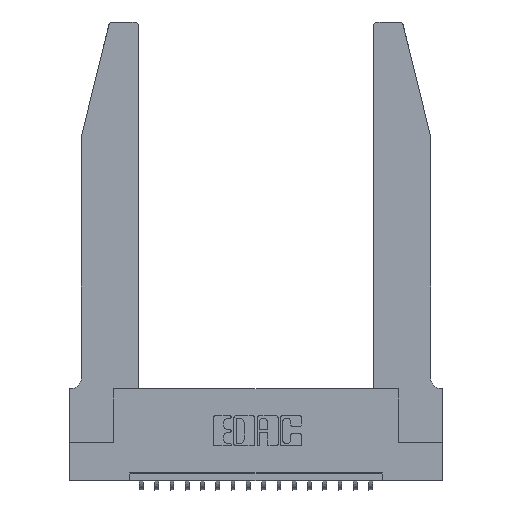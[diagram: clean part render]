
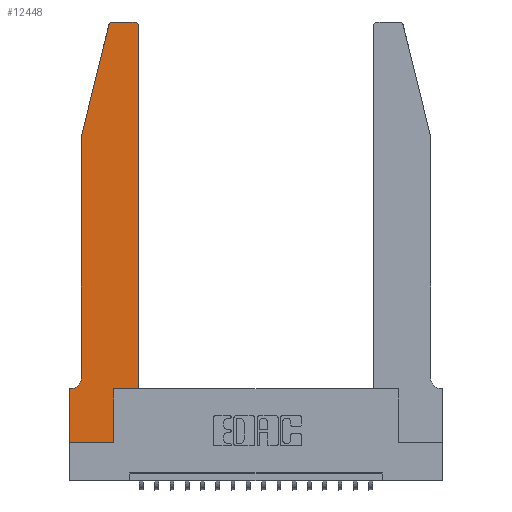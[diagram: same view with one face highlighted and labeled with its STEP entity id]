
A CAD part, top view. The second image highlights one B-rep face of the part: STEP entity #12448.
In plain terms, the highlighted planar face has unit normal (0, 0, 1).
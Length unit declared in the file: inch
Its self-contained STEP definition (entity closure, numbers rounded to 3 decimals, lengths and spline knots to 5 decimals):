
#5 = VECTOR ( 'NONE', #10087, 39.37008 ) ;
#190 = CARTESIAN_POINT ( 'NONE',  ( 0.2865, 0., 0.37 ) ) ;
#705 = LINE ( 'NONE', #11188, #4905 ) ;
#802 = FACE_OUTER_BOUND ( 'NONE', #14091, .T. ) ;
#863 = VERTEX_POINT ( 'NONE', #9467 ) ;
#994 = VECTOR ( 'NONE', #8657, 39.37008 ) ;
#1489 = CARTESIAN_POINT ( 'NONE',  ( 0.4505, 0.35, 0.37 ) ) ;
#1518 = CARTESIAN_POINT ( 'NONE',  ( 0.0755, 2., 0.37 ) ) ;
#1548 = ORIENTED_EDGE ( 'NONE', *, *, #9889, .T. ) ;
#1733 = VERTEX_POINT ( 'NONE', #190 ) ;
#1783 = EDGE_CURVE ( 'NONE', #2787, #863, #7166, .T. ) ;
#2055 = CIRCLE ( 'NONE', #8243, 0.03 ) ;
#2124 = EDGE_CURVE ( 'NONE', #19812, #16952, #705, .T. ) ;
#2198 = CARTESIAN_POINT ( 'NONE',  ( 0.0755, 2., 0.37 ) ) ;
#2612 = EDGE_CURVE ( 'NONE', #8820, #2787, #18399, .T. ) ;
#2787 = VERTEX_POINT ( 'NONE', #7991 ) ;
#3136 = LINE ( 'NONE', #4135, #8361 ) ;
#3160 = VECTOR ( 'NONE', #18661, 39.37008 ) ;
#3283 = DIRECTION ( 'NONE',  ( 0., 0., 1. ) ) ;
#3420 = DIRECTION ( 'NONE',  ( 1., 0., 0. ) ) ;
#3585 = VECTOR ( 'NONE', #6694, 39.37008 ) ;
#3654 = CARTESIAN_POINT ( 'NONE',  ( 0., 0., 0.37 ) ) ;
#3761 = CARTESIAN_POINT ( 'NONE',  ( 0.4505, 2.72, 0.37 ) ) ;
#3917 = CARTESIAN_POINT ( 'NONE',  ( 0., 0.35, 0.37 ) ) ;
#4112 = ORIENTED_EDGE ( 'NONE', *, *, #6686, .T. ) ;
#4135 = CARTESIAN_POINT ( 'NONE',  ( 0.4505, 0.35, 0.37 ) ) ;
#4339 = DIRECTION ( 'NONE',  ( 0., 1., 0. ) ) ;
#4411 = ORIENTED_EDGE ( 'NONE', *, *, #4418, .T. ) ;
#4416 = VECTOR ( 'NONE', #17747, 39.37008 ) ;
#4418 = EDGE_CURVE ( 'NONE', #6500, #11120, #15880, .T. ) ;
#4796 = LINE ( 'NONE', #2198, #3585 ) ;
#4838 = ORIENTED_EDGE ( 'NONE', *, *, #2124, .T. ) ;
#4905 = VECTOR ( 'NONE', #19212, 39.37008 ) ;
#5016 = VERTEX_POINT ( 'NONE', #18807 ) ;
#5957 = LINE ( 'NONE', #20097, #15311 ) ;
#6092 = AXIS2_PLACEMENT_3D ( 'NONE', #3917, #14924, #6916 ) ;
#6423 = ORIENTED_EDGE ( 'NONE', *, *, #8244, .T. ) ;
#6500 = VERTEX_POINT ( 'NONE', #10974 ) ;
#6686 = EDGE_CURVE ( 'NONE', #8183, #9605, #6714, .T. ) ;
#6694 = DIRECTION ( 'NONE',  ( 0., -1., 0. ) ) ;
#6714 = LINE ( 'NONE', #14637, #994 ) ;
#6756 = EDGE_CURVE ( 'NONE', #863, #1733, #13086, .T. ) ;
#6905 = EDGE_CURVE ( 'NONE', #1733, #6500, #5957, .T. ) ;
#6916 = DIRECTION ( 'NONE',  ( 1., 0., 0. ) ) ;
#7166 = LINE ( 'NONE', #3654, #4416 ) ;
#7494 = ORIENTED_EDGE ( 'NONE', *, *, #2612, .T. ) ;
#7991 = CARTESIAN_POINT ( 'NONE',  ( 0., 0.35, 0.37 ) ) ;
#8005 = CARTESIAN_POINT ( 'NONE',  ( 0.284, 2.72, 0.37 ) ) ;
#8081 = CARTESIAN_POINT ( 'NONE',  ( 0.4205, 2.75, 0.37 ) ) ;
#8183 = VERTEX_POINT ( 'NONE', #8081 ) ;
#8243 = AXIS2_PLACEMENT_3D ( 'NONE', #14867, #13280, #19529 ) ;
#8244 = EDGE_CURVE ( 'NONE', #5016, #8820, #9862, .T. ) ;
#8361 = VECTOR ( 'NONE', #4339, 39.37008 ) ;
#8657 = DIRECTION ( 'NONE',  ( -1., 0., 0. ) ) ;
#8820 = VERTEX_POINT ( 'NONE', #11243 ) ;
#9307 = DIRECTION ( 'NONE',  ( 0., 1., 0. ) ) ;
#9467 = CARTESIAN_POINT ( 'NONE',  ( 0., 0., 0.37 ) ) ;
#9543 = DIRECTION ( 'NONE',  ( 1., 0., 0. ) ) ;
#9605 = VERTEX_POINT ( 'NONE', #20060 ) ;
#9862 = CIRCLE ( 'NONE', #12224, 0.07 ) ;
#9889 = EDGE_CURVE ( 'NONE', #9605, #19812, #19123, .T. ) ;
#10087 = DIRECTION ( 'NONE',  ( 1., 0., 0. ) ) ;
#10127 = ORIENTED_EDGE ( 'NONE', *, *, #18712, .T. ) ;
#10186 = PLANE ( 'NONE',  #6092 ) ;
#10449 = VECTOR ( 'NONE', #9543, 39.37008 ) ;
#10974 = CARTESIAN_POINT ( 'NONE',  ( 0.2865, 0.35, 0.37 ) ) ;
#11084 = CARTESIAN_POINT ( 'NONE',  ( 0.25487, 2.72718, 0.37 ) ) ;
#11120 = VERTEX_POINT ( 'NONE', #16095 ) ;
#11184 = EDGE_CURVE ( 'NONE', #16952, #5016, #4796, .T. ) ;
#11188 = CARTESIAN_POINT ( 'NONE',  ( 0.0755, 2., 0.37 ) ) ;
#11243 = CARTESIAN_POINT ( 'NONE',  ( 0.0055, 0.35, 0.37 ) ) ;
#11437 = DIRECTION ( 'NONE',  ( 0., 0., -1. ) ) ;
#12224 = AXIS2_PLACEMENT_3D ( 'NONE', #15900, #11437, #14593 ) ;
#12282 = ORIENTED_EDGE ( 'NONE', *, *, #6756, .T. ) ;
#12448 = ADVANCED_FACE ( 'NONE', ( #802 ), #10186, .T. ) ;
#12502 = EDGE_CURVE ( 'NONE', #16379, #8183, #2055, .T. ) ;
#13086 = LINE ( 'NONE', #16406, #5 ) ;
#13280 = DIRECTION ( 'NONE',  ( 0., 0., 1. ) ) ;
#13624 = ORIENTED_EDGE ( 'NONE', *, *, #6905, .T. ) ;
#14091 = EDGE_LOOP ( 'NONE', ( #4112, #1548, #4838, #15078, #6423, #7494, #15122, #12282, #13624, #4411, #10127, #16305 ) ) ;
#14593 = DIRECTION ( 'NONE',  ( -1., 0., 0. ) ) ;
#14637 = CARTESIAN_POINT ( 'NONE',  ( 0.2605, 2.75, 0.37 ) ) ;
#14867 = CARTESIAN_POINT ( 'NONE',  ( 0.4205, 2.72, 0.37 ) ) ;
#14924 = DIRECTION ( 'NONE',  ( 0., 0., 1. ) ) ;
#15078 = ORIENTED_EDGE ( 'NONE', *, *, #11184, .T. ) ;
#15122 = ORIENTED_EDGE ( 'NONE', *, *, #1783, .T. ) ;
#15311 = VECTOR ( 'NONE', #9307, 39.37008 ) ;
#15880 = LINE ( 'NONE', #1489, #10449 ) ;
#15900 = CARTESIAN_POINT ( 'NONE',  ( 0.0055, 0.42, 0.37 ) ) ;
#16095 = CARTESIAN_POINT ( 'NONE',  ( 0.4505, 0.35, 0.37 ) ) ;
#16305 = ORIENTED_EDGE ( 'NONE', *, *, #12502, .T. ) ;
#16327 = AXIS2_PLACEMENT_3D ( 'NONE', #8005, #3283, #3420 ) ;
#16379 = VERTEX_POINT ( 'NONE', #3761 ) ;
#16406 = CARTESIAN_POINT ( 'NONE',  ( 0., 0., 0.37 ) ) ;
#16952 = VERTEX_POINT ( 'NONE', #1518 ) ;
#17747 = DIRECTION ( 'NONE',  ( 0., -1., 0. ) ) ;
#18399 = LINE ( 'NONE', #18455, #3160 ) ;
#18455 = CARTESIAN_POINT ( 'NONE',  ( 0.0755, 0.35, 0.37 ) ) ;
#18661 = DIRECTION ( 'NONE',  ( -1., 0., 0. ) ) ;
#18712 = EDGE_CURVE ( 'NONE', #11120, #16379, #3136, .T. ) ;
#18807 = CARTESIAN_POINT ( 'NONE',  ( 0.0755, 0.42, 0.37 ) ) ;
#19123 = CIRCLE ( 'NONE', #16327, 0.03 ) ;
#19212 = DIRECTION ( 'NONE',  ( -0.239, -0.971, 0. ) ) ;
#19529 = DIRECTION ( 'NONE',  ( 1., 0., 0. ) ) ;
#19812 = VERTEX_POINT ( 'NONE', #11084 ) ;
#20060 = CARTESIAN_POINT ( 'NONE',  ( 0.284, 2.75, 0.37 ) ) ;
#20097 = CARTESIAN_POINT ( 'NONE',  ( 0.2865, 0.35, 0.37 ) ) ;
